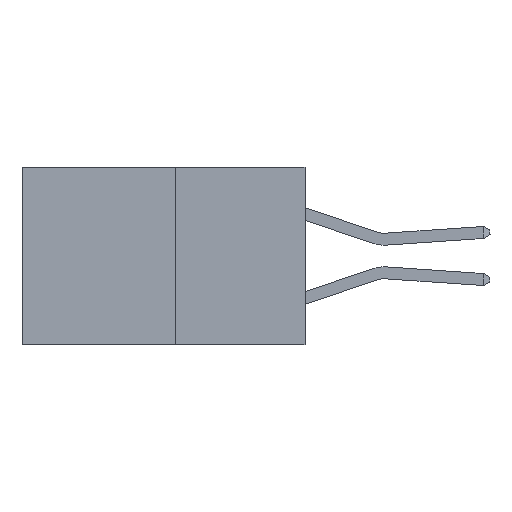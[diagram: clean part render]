
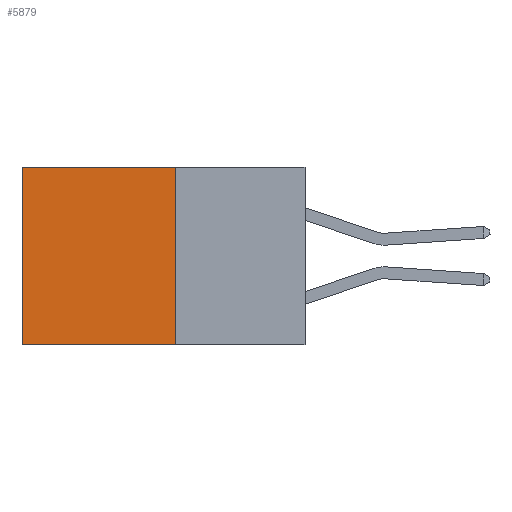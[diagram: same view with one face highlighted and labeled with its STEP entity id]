
A CAD part, left-side view. The second image highlights one B-rep face of the part: STEP entity #5879.
In plain terms, the highlighted planar face has unit normal (-1, 0, 0).
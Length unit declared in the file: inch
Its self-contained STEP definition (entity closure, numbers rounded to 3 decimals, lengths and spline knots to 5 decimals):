
#1580 = PLANE ( 'NONE',  #25443 ) ;
#3037 = VERTEX_POINT ( 'NONE', #5696 ) ;
#3176 = LINE ( 'NONE', #8772, #19309 ) ;
#3781 = CARTESIAN_POINT ( 'NONE',  ( 0.277, 0.27, -0.37 ) ) ;
#4445 = CARTESIAN_POINT ( 'NONE',  ( 0.277, 0.59, -0.37 ) ) ;
#5696 = CARTESIAN_POINT ( 'NONE',  ( 0.277, 0.59, 0. ) ) ;
#5791 = CARTESIAN_POINT ( 'NONE',  ( 0.277, 0.27, -0.37 ) ) ;
#5879 = ADVANCED_FACE ( 'NONE', ( #23525 ), #1580, .F. ) ;
#5950 = DIRECTION ( 'NONE',  ( 1., 0., 0. ) ) ;
#7924 = DIRECTION ( 'NONE',  ( 0., 1., 0. ) ) ;
#8772 = CARTESIAN_POINT ( 'NONE',  ( 0.277, 0.27, 0. ) ) ;
#8996 = LINE ( 'NONE', #27068, #18129 ) ;
#9508 = ORIENTED_EDGE ( 'NONE', *, *, #10902, .F. ) ;
#9699 = EDGE_CURVE ( 'NONE', #3037, #23111, #23978, .T. ) ;
#10004 = CARTESIAN_POINT ( 'NONE',  ( 0.277, 0.59, -0.37 ) ) ;
#10147 = VERTEX_POINT ( 'NONE', #18175 ) ;
#10294 = LINE ( 'NONE', #5791, #15206 ) ;
#10310 = ORIENTED_EDGE ( 'NONE', *, *, #9699, .T. ) ;
#10320 = EDGE_CURVE ( 'NONE', #10147, #23844, #8996, .T. ) ;
#10902 = EDGE_CURVE ( 'NONE', #23844, #23111, #10294, .T. ) ;
#10910 = DIRECTION ( 'NONE',  ( 0., 1., 0. ) ) ;
#11030 = ORIENTED_EDGE ( 'NONE', *, *, #10320, .F. ) ;
#13176 = EDGE_CURVE ( 'NONE', #10147, #3037, #3176, .T. ) ;
#15206 = VECTOR ( 'NONE', #7924, 39.37008 ) ;
#15884 = ORIENTED_EDGE ( 'NONE', *, *, #13176, .T. ) ;
#17027 = DIRECTION ( 'NONE',  ( 0., 0., -1. ) ) ;
#18129 = VECTOR ( 'NONE', #22934, 39.37008 ) ;
#18175 = CARTESIAN_POINT ( 'NONE',  ( 0.277, 0.27, 0. ) ) ;
#19309 = VECTOR ( 'NONE', #10910, 39.37008 ) ;
#20561 = DIRECTION ( 'NONE',  ( 0., 0., -1. ) ) ;
#22669 = VECTOR ( 'NONE', #17027, 39.37008 ) ;
#22934 = DIRECTION ( 'NONE',  ( 0., 0., -1. ) ) ;
#23039 = CARTESIAN_POINT ( 'NONE',  ( 0.277, 0.27, -0.37 ) ) ;
#23111 = VERTEX_POINT ( 'NONE', #10004 ) ;
#23525 = FACE_OUTER_BOUND ( 'NONE', #26845, .T. ) ;
#23844 = VERTEX_POINT ( 'NONE', #23039 ) ;
#23978 = LINE ( 'NONE', #4445, #22669 ) ;
#25443 = AXIS2_PLACEMENT_3D ( 'NONE', #3781, #5950, #20561 ) ;
#26845 = EDGE_LOOP ( 'NONE', ( #10310, #9508, #11030, #15884 ) ) ;
#27068 = CARTESIAN_POINT ( 'NONE',  ( 0.277, 0.27, -0.37 ) ) ;
